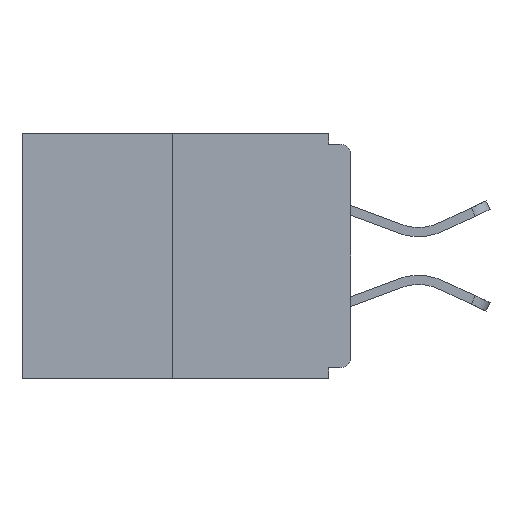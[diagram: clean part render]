
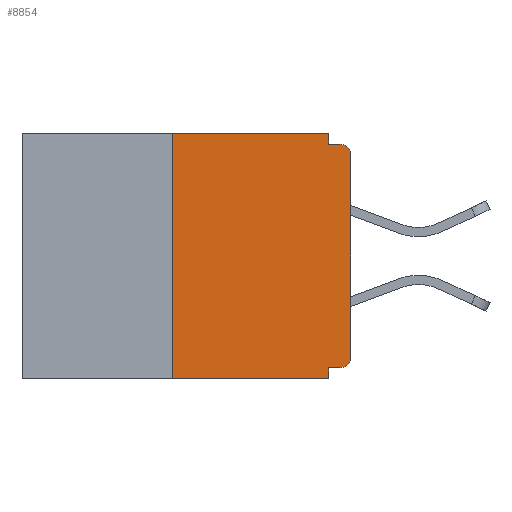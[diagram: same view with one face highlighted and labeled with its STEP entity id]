
A CAD part, left-side view. The second image highlights one B-rep face of the part: STEP entity #8854.
In plain terms, the highlighted planar face has unit normal (-1, 0, 0).
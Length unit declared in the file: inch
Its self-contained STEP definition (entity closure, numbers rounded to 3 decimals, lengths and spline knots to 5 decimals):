
#387 = EDGE_CURVE ( 'NONE', #12959, #2673, #5474, .T. ) ;
#597 = ORIENTED_EDGE ( 'NONE', *, *, #3514, .T. ) ;
#754 = LINE ( 'NONE', #11898, #8598 ) ;
#1190 = ORIENTED_EDGE ( 'NONE', *, *, #9613, .F. ) ;
#1206 = CARTESIAN_POINT ( 'NONE',  ( 0., 0., -0.328 ) ) ;
#1247 = DIRECTION ( 'NONE',  ( 0., 0., -1. ) ) ;
#1321 = DIRECTION ( 'NONE',  ( 0., -1., 0. ) ) ;
#1695 = VECTOR ( 'NONE', #13051, 39.37008 ) ;
#1781 = CARTESIAN_POINT ( 'NONE',  ( 0., 0.031, 0. ) ) ;
#1833 = CARTESIAN_POINT ( 'NONE',  ( 0., 0.46, -0.343 ) ) ;
#2142 = CIRCLE ( 'NONE', #7773, 0.015 ) ;
#2174 = EDGE_LOOP ( 'NONE', ( #14312, #1190, #16628, #7820, #5892, #4884, #597, #15922, #15312, #3043 ) ) ;
#2590 = EDGE_CURVE ( 'NONE', #2673, #14656, #10710, .T. ) ;
#2673 = VERTEX_POINT ( 'NONE', #15508 ) ;
#3015 = CARTESIAN_POINT ( 'NONE',  ( 0., 0.015, -0.328 ) ) ;
#3043 = ORIENTED_EDGE ( 'NONE', *, *, #13455, .F. ) ;
#3122 = VERTEX_POINT ( 'NONE', #5336 ) ;
#3123 = DIRECTION ( 'NONE',  ( 0., 0., -1. ) ) ;
#3514 = EDGE_CURVE ( 'NONE', #13362, #11161, #7763, .T. ) ;
#3770 = DIRECTION ( 'NONE',  ( 0., 0., -1. ) ) ;
#3969 = EDGE_CURVE ( 'NONE', #16866, #13670, #16451, .T. ) ;
#4183 = DIRECTION ( 'NONE',  ( 0., -1., 0. ) ) ;
#4227 = FACE_OUTER_BOUND ( 'NONE', #2174, .T. ) ;
#4499 = VECTOR ( 'NONE', #1321, 39.37008 ) ;
#4523 = DIRECTION ( 'NONE',  ( -1., 0., 0. ) ) ;
#4828 = CARTESIAN_POINT ( 'NONE',  ( 0., 0., -0.03 ) ) ;
#4884 = ORIENTED_EDGE ( 'NONE', *, *, #5806, .T. ) ;
#5120 = CARTESIAN_POINT ( 'NONE',  ( 0., 0.25, 0. ) ) ;
#5336 = CARTESIAN_POINT ( 'NONE',  ( 0., 0.015, -0.015 ) ) ;
#5474 = LINE ( 'NONE', #1206, #9997 ) ;
#5546 = DIRECTION ( 'NONE',  ( -1., 0., 0. ) ) ;
#5712 = VECTOR ( 'NONE', #14419, 39.37008 ) ;
#5806 = EDGE_CURVE ( 'NONE', #12959, #13362, #2142, .T. ) ;
#5892 = ORIENTED_EDGE ( 'NONE', *, *, #387, .F. ) ;
#6452 = CARTESIAN_POINT ( 'NONE',  ( 0., 0.031, -0.343 ) ) ;
#6906 = DIRECTION ( 'NONE',  ( 0., 0., -1. ) ) ;
#7603 = CIRCLE ( 'NONE', #14766, 0.015 ) ;
#7763 = LINE ( 'NONE', #12730, #12963 ) ;
#7773 = AXIS2_PLACEMENT_3D ( 'NONE', #13511, #5546, #3123 ) ;
#7820 = ORIENTED_EDGE ( 'NONE', *, *, #2590, .F. ) ;
#7828 = CARTESIAN_POINT ( 'NONE',  ( 0., 0.015, -0.03 ) ) ;
#8293 = CARTESIAN_POINT ( 'NONE',  ( 0., 0.46, 0. ) ) ;
#8598 = VECTOR ( 'NONE', #3770, 39.37008 ) ;
#8667 = DIRECTION ( 'NONE',  ( 0., 0., 1. ) ) ;
#8854 = ADVANCED_FACE ( 'NONE', ( #4227 ), #14921, .F. ) ;
#8939 = AXIS2_PLACEMENT_3D ( 'NONE', #8293, #13615, #6906 ) ;
#9613 = EDGE_CURVE ( 'NONE', #15757, #16866, #16376, .T. ) ;
#9997 = VECTOR ( 'NONE', #10434, 39.37008 ) ;
#10285 = VECTOR ( 'NONE', #1247, 39.37008 ) ;
#10434 = DIRECTION ( 'NONE',  ( 0., 1., 0. ) ) ;
#10710 = LINE ( 'NONE', #6452, #10285 ) ;
#11161 = VERTEX_POINT ( 'NONE', #4828 ) ;
#11868 = VERTEX_POINT ( 'NONE', #15401 ) ;
#11898 = CARTESIAN_POINT ( 'NONE',  ( 0., 0.031, 0. ) ) ;
#11908 = EDGE_CURVE ( 'NONE', #11161, #3122, #7603, .T. ) ;
#12132 = LINE ( 'NONE', #1833, #4499 ) ;
#12730 = CARTESIAN_POINT ( 'NONE',  ( 0., 0., 0. ) ) ;
#12959 = VERTEX_POINT ( 'NONE', #3015 ) ;
#12963 = VECTOR ( 'NONE', #8667, 39.37008 ) ;
#13051 = DIRECTION ( 'NONE',  ( 0., 0., 1. ) ) ;
#13232 = CARTESIAN_POINT ( 'NONE',  ( 0., 0., -0.015 ) ) ;
#13362 = VERTEX_POINT ( 'NONE', #17019 ) ;
#13395 = CARTESIAN_POINT ( 'NONE',  ( 0., 0.25, -0.343 ) ) ;
#13440 = EDGE_CURVE ( 'NONE', #15757, #14656, #12132, .T. ) ;
#13455 = EDGE_CURVE ( 'NONE', #13670, #11868, #754, .T. ) ;
#13511 = CARTESIAN_POINT ( 'NONE',  ( 0., 0.015, -0.313 ) ) ;
#13550 = CARTESIAN_POINT ( 'NONE',  ( 0., 0.25, 0. ) ) ;
#13615 = DIRECTION ( 'NONE',  ( 1., 0., 0. ) ) ;
#13670 = VERTEX_POINT ( 'NONE', #1781 ) ;
#14312 = ORIENTED_EDGE ( 'NONE', *, *, #3969, .F. ) ;
#14386 = VECTOR ( 'NONE', #4183, 39.37008 ) ;
#14419 = DIRECTION ( 'NONE',  ( 0., -1., 0. ) ) ;
#14460 = EDGE_CURVE ( 'NONE', #11868, #3122, #14792, .T. ) ;
#14656 = VERTEX_POINT ( 'NONE', #15427 ) ;
#14717 = CARTESIAN_POINT ( 'NONE',  ( 0., 0.46, 0. ) ) ;
#14766 = AXIS2_PLACEMENT_3D ( 'NONE', #7828, #4523, #17015 ) ;
#14792 = LINE ( 'NONE', #13232, #5712 ) ;
#14921 = PLANE ( 'NONE',  #8939 ) ;
#15312 = ORIENTED_EDGE ( 'NONE', *, *, #14460, .F. ) ;
#15401 = CARTESIAN_POINT ( 'NONE',  ( 0., 0.031, -0.015 ) ) ;
#15427 = CARTESIAN_POINT ( 'NONE',  ( 0., 0.031, -0.343 ) ) ;
#15508 = CARTESIAN_POINT ( 'NONE',  ( 0., 0.031, -0.328 ) ) ;
#15757 = VERTEX_POINT ( 'NONE', #13395 ) ;
#15922 = ORIENTED_EDGE ( 'NONE', *, *, #11908, .T. ) ;
#16376 = LINE ( 'NONE', #5120, #1695 ) ;
#16451 = LINE ( 'NONE', #14717, #14386 ) ;
#16628 = ORIENTED_EDGE ( 'NONE', *, *, #13440, .T. ) ;
#16866 = VERTEX_POINT ( 'NONE', #13550 ) ;
#17015 = DIRECTION ( 'NONE',  ( 0., 0., -1. ) ) ;
#17019 = CARTESIAN_POINT ( 'NONE',  ( 0., 0., -0.313 ) ) ;
